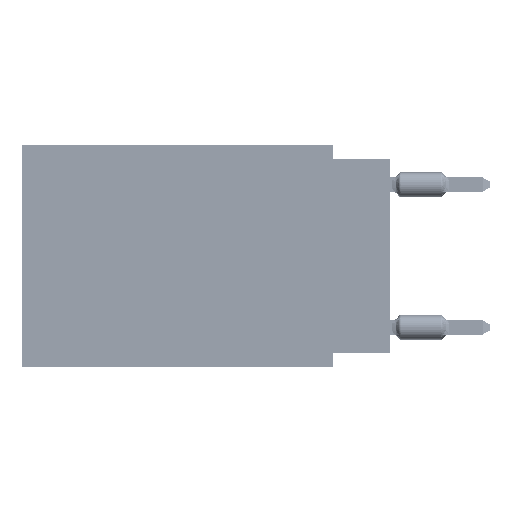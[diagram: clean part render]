
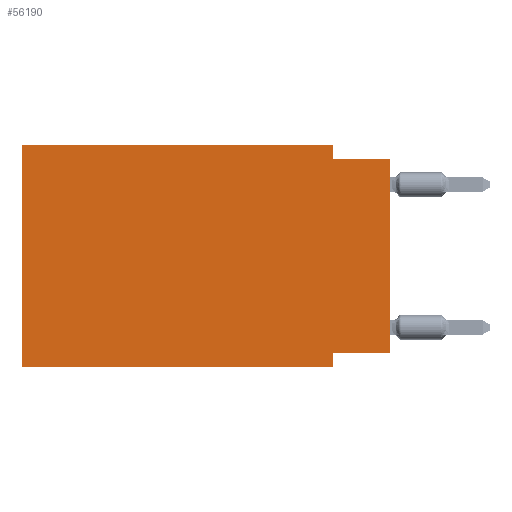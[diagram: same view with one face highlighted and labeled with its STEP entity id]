
A CAD part, left-side view. The second image highlights one B-rep face of the part: STEP entity #56190.
In plain terms, the highlighted planar face has unit normal (-1, 0, 0).
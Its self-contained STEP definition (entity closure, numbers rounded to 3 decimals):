
#312 = VECTOR ( 'NONE', #22866, 1000. ) ;
#721 = DIRECTION ( 'NONE',  ( 0., -1., 0. ) ) ;
#880 = AXIS2_PLACEMENT_3D ( 'NONE', #48990, #65760, #17846 ) ;
#1266 = EDGE_CURVE ( 'NONE', #14504, #34242, #21752, .T. ) ;
#3684 = DIRECTION ( 'NONE',  ( 0., 0., 1. ) ) ;
#5135 = ORIENTED_EDGE ( 'NONE', *, *, #10546, .T. ) ;
#6590 = DIRECTION ( 'NONE',  ( 0., 0., -1. ) ) ;
#9648 = LINE ( 'NONE', #33984, #23543 ) ;
#10546 = EDGE_CURVE ( 'NONE', #38864, #55143, #9648, .T. ) ;
#12121 = CARTESIAN_POINT ( 'NONE',  ( 0., 0., -9.271 ) ) ;
#12964 = LINE ( 'NONE', #66837, #69030 ) ;
#14246 = EDGE_CURVE ( 'NONE', #60121, #55143, #22878, .T. ) ;
#14504 = VERTEX_POINT ( 'NONE', #15993 ) ;
#14979 = CARTESIAN_POINT ( 'NONE',  ( 0., 16.383, 0. ) ) ;
#15993 = CARTESIAN_POINT ( 'NONE',  ( 0., 16.383, 0. ) ) ;
#16898 = VECTOR ( 'NONE', #721, 1000. ) ;
#17271 = DIRECTION ( 'NONE',  ( 0., -1., 0. ) ) ;
#17732 = DIRECTION ( 'NONE',  ( 0., -1., 0. ) ) ;
#17846 = DIRECTION ( 'NONE',  ( 0., 0., -1. ) ) ;
#18945 = CARTESIAN_POINT ( 'NONE',  ( 0., 2.54, -9.906 ) ) ;
#19491 = CARTESIAN_POINT ( 'NONE',  ( 0., 2.54, 0. ) ) ;
#20210 = ORIENTED_EDGE ( 'NONE', *, *, #69738, .F. ) ;
#21126 = VECTOR ( 'NONE', #48073, 1000. ) ;
#21752 = LINE ( 'NONE', #28148, #68509 ) ;
#22024 = CARTESIAN_POINT ( 'NONE',  ( 0., 2.54, -0.635 ) ) ;
#22189 = EDGE_CURVE ( 'NONE', #38864, #37334, #23642, .T. ) ;
#22866 = DIRECTION ( 'NONE',  ( 0., 1., 0. ) ) ;
#22878 = LINE ( 'NONE', #47234, #71174 ) ;
#23543 = VECTOR ( 'NONE', #3684, 1000. ) ;
#23642 = LINE ( 'NONE', #40833, #312 ) ;
#23708 = ORIENTED_EDGE ( 'NONE', *, *, #68516, .F. ) ;
#28148 = CARTESIAN_POINT ( 'NONE',  ( 0., 16.383, 0. ) ) ;
#29698 = LINE ( 'NONE', #41292, #21126 ) ;
#30038 = ORIENTED_EDGE ( 'NONE', *, *, #72474, .F. ) ;
#33984 = CARTESIAN_POINT ( 'NONE',  ( 0., 0., 0. ) ) ;
#34222 = VERTEX_POINT ( 'NONE', #74171 ) ;
#34242 = VERTEX_POINT ( 'NONE', #19491 ) ;
#36217 = PLANE ( 'NONE',  #880 ) ;
#37334 = VERTEX_POINT ( 'NONE', #38613 ) ;
#37355 = ORIENTED_EDGE ( 'NONE', *, *, #22189, .F. ) ;
#37736 = ORIENTED_EDGE ( 'NONE', *, *, #73278, .T. ) ;
#38613 = CARTESIAN_POINT ( 'NONE',  ( 0., 2.54, -9.271 ) ) ;
#38864 = VERTEX_POINT ( 'NONE', #12121 ) ;
#39349 = DIRECTION ( 'NONE',  ( 0., 0., 1. ) ) ;
#40833 = CARTESIAN_POINT ( 'NONE',  ( 0., 0., -9.271 ) ) ;
#41292 = CARTESIAN_POINT ( 'NONE',  ( 0., 2.54, -9.906 ) ) ;
#47234 = CARTESIAN_POINT ( 'NONE',  ( 0., 0., -0.635 ) ) ;
#48073 = DIRECTION ( 'NONE',  ( 0., 0., -1. ) ) ;
#48990 = CARTESIAN_POINT ( 'NONE',  ( 0., 16.383, 0. ) ) ;
#55143 = VERTEX_POINT ( 'NONE', #58392 ) ;
#55382 = LINE ( 'NONE', #74108, #16898 ) ;
#56190 = ADVANCED_FACE ( 'NONE', ( #72521 ), #36217, .F. ) ;
#58392 = CARTESIAN_POINT ( 'NONE',  ( 0., 0., -0.635 ) ) ;
#60121 = VERTEX_POINT ( 'NONE', #22024 ) ;
#64851 = EDGE_LOOP ( 'NONE', ( #5135, #74094, #30038, #74880, #20210, #37736, #23708, #37355 ) ) ;
#65760 = DIRECTION ( 'NONE',  ( 1., 0., 0. ) ) ;
#66837 = CARTESIAN_POINT ( 'NONE',  ( 0., 2.54, 0. ) ) ;
#67538 = VECTOR ( 'NONE', #39349, 1000. ) ;
#68509 = VECTOR ( 'NONE', #17732, 1000. ) ;
#68516 = EDGE_CURVE ( 'NONE', #37334, #72512, #29698, .T. ) ;
#69030 = VECTOR ( 'NONE', #6590, 1000. ) ;
#69652 = LINE ( 'NONE', #14979, #67538 ) ;
#69738 = EDGE_CURVE ( 'NONE', #34222, #14504, #69652, .T. ) ;
#71174 = VECTOR ( 'NONE', #17271, 1000. ) ;
#72474 = EDGE_CURVE ( 'NONE', #34242, #60121, #12964, .T. ) ;
#72512 = VERTEX_POINT ( 'NONE', #18945 ) ;
#72521 = FACE_OUTER_BOUND ( 'NONE', #64851, .T. ) ;
#73278 = EDGE_CURVE ( 'NONE', #34222, #72512, #55382, .T. ) ;
#74094 = ORIENTED_EDGE ( 'NONE', *, *, #14246, .F. ) ;
#74108 = CARTESIAN_POINT ( 'NONE',  ( 0., 16.383, -9.906 ) ) ;
#74171 = CARTESIAN_POINT ( 'NONE',  ( 0., 16.383, -9.906 ) ) ;
#74880 = ORIENTED_EDGE ( 'NONE', *, *, #1266, .F. ) ;
